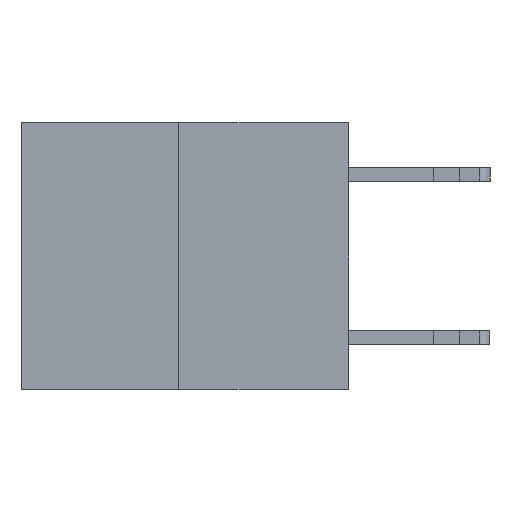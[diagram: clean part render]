
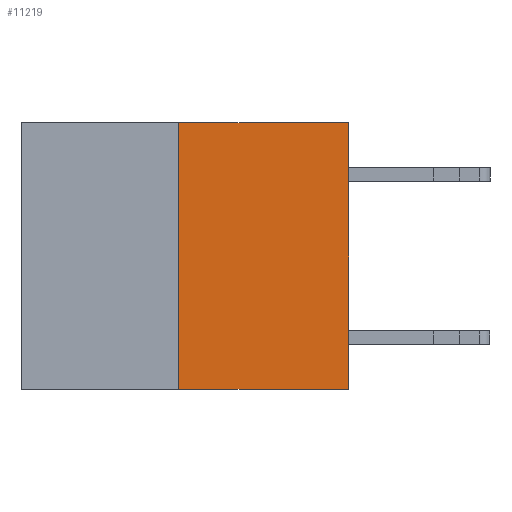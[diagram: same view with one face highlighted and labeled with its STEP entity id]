
A CAD part, left-side view. The second image highlights one B-rep face of the part: STEP entity #11219.
In plain terms, the highlighted planar face has unit normal (-1, 0, 0).
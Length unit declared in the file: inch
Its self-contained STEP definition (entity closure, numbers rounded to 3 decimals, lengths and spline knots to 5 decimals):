
#140 = VECTOR ( 'NONE', #9595, 39.37008 ) ;
#531 = VERTEX_POINT ( 'NONE', #5691 ) ;
#899 = VERTEX_POINT ( 'NONE', #7518 ) ;
#1008 = DIRECTION ( 'NONE',  ( 0., 0., 1. ) ) ;
#1061 = ORIENTED_EDGE ( 'NONE', *, *, #8348, .T. ) ;
#1415 = VERTEX_POINT ( 'NONE', #4976 ) ;
#2399 = DIRECTION ( 'NONE',  ( 0., 0., -1. ) ) ;
#4976 = CARTESIAN_POINT ( 'NONE',  ( 0., 0.312, -0.49 ) ) ;
#5430 = LINE ( 'NONE', #6399, #6256 ) ;
#5691 = CARTESIAN_POINT ( 'NONE',  ( 0., 0., -0.49 ) ) ;
#6047 = EDGE_LOOP ( 'NONE', ( #12965, #1061, #14276, #7810 ) ) ;
#6145 = EDGE_CURVE ( 'NONE', #9485, #899, #11467, .T. ) ;
#6256 = VECTOR ( 'NONE', #12973, 39.37008 ) ;
#6399 = CARTESIAN_POINT ( 'NONE',  ( 0., 0.6, -0.49 ) ) ;
#6598 = VECTOR ( 'NONE', #1008, 39.37008 ) ;
#7138 = AXIS2_PLACEMENT_3D ( 'NONE', #12719, #15427, #2399 ) ;
#7518 = CARTESIAN_POINT ( 'NONE',  ( 0., 0., 0. ) ) ;
#7612 = FACE_OUTER_BOUND ( 'NONE', #6047, .T. ) ;
#7810 = ORIENTED_EDGE ( 'NONE', *, *, #6145, .F. ) ;
#8348 = EDGE_CURVE ( 'NONE', #1415, #531, #5430, .T. ) ;
#8737 = PLANE ( 'NONE',  #7138 ) ;
#9465 = DIRECTION ( 'NONE',  ( 0., -1., 0. ) ) ;
#9485 = VERTEX_POINT ( 'NONE', #11372 ) ;
#9595 = DIRECTION ( 'NONE',  ( 0., 0., 1. ) ) ;
#9710 = CARTESIAN_POINT ( 'NONE',  ( 0., 0., 0. ) ) ;
#9916 = EDGE_CURVE ( 'NONE', #1415, #9485, #14375, .T. ) ;
#11219 = ADVANCED_FACE ( 'NONE', ( #7612 ), #8737, .F. ) ;
#11372 = CARTESIAN_POINT ( 'NONE',  ( 0., 0.312, 0. ) ) ;
#11467 = LINE ( 'NONE', #13526, #14492 ) ;
#12719 = CARTESIAN_POINT ( 'NONE',  ( 0., 0.6, 0. ) ) ;
#12965 = ORIENTED_EDGE ( 'NONE', *, *, #9916, .F. ) ;
#12973 = DIRECTION ( 'NONE',  ( 0., -1., 0. ) ) ;
#13526 = CARTESIAN_POINT ( 'NONE',  ( 0., 0.6, 0. ) ) ;
#14276 = ORIENTED_EDGE ( 'NONE', *, *, #15376, .T. ) ;
#14375 = LINE ( 'NONE', #16802, #6598 ) ;
#14492 = VECTOR ( 'NONE', #9465, 39.37008 ) ;
#15376 = EDGE_CURVE ( 'NONE', #531, #899, #15621, .T. ) ;
#15427 = DIRECTION ( 'NONE',  ( 1., 0., 0. ) ) ;
#15621 = LINE ( 'NONE', #9710, #140 ) ;
#16802 = CARTESIAN_POINT ( 'NONE',  ( 0., 0.312, -0.49 ) ) ;
